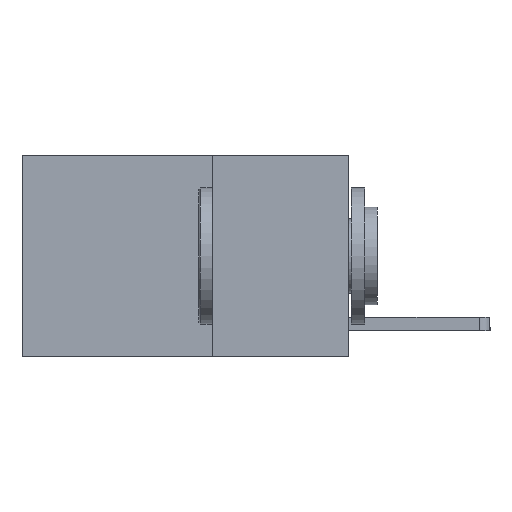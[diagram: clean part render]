
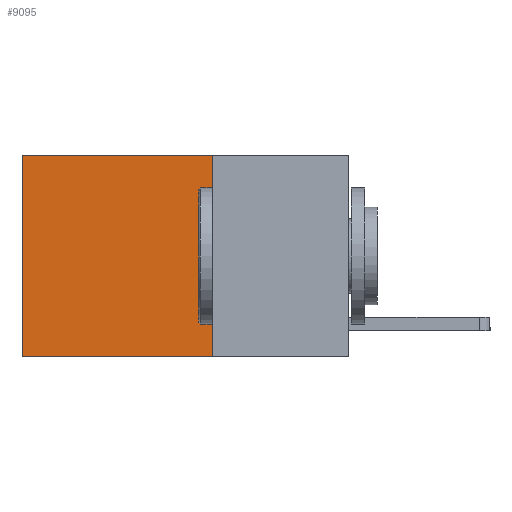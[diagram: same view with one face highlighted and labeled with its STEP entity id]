
A CAD part, left-side view. The second image highlights one B-rep face of the part: STEP entity #9095.
In plain terms, the highlighted planar face has unit normal (-1, 0, 0).
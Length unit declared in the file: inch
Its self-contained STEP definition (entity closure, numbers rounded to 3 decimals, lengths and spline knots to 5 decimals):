
#78 = VECTOR ( 'NONE', #3506, 39.37008 ) ;
#290 = EDGE_CURVE ( 'NONE', #3493, #10487, #9896, .T. ) ;
#1287 = ORIENTED_EDGE ( 'NONE', *, *, #3142, .T. ) ;
#1579 = AXIS2_PLACEMENT_3D ( 'NONE', #5952, #8208, #4128 ) ;
#2657 = VECTOR ( 'NONE', #7800, 39.37008 ) ;
#3085 = EDGE_LOOP ( 'NONE', ( #1287, #8092, #6186, #6902 ) ) ;
#3142 = EDGE_CURVE ( 'NONE', #10487, #8036, #9861, .T. ) ;
#3428 = PLANE ( 'NONE',  #1579 ) ;
#3493 = VERTEX_POINT ( 'NONE', #7069 ) ;
#3506 = DIRECTION ( 'NONE',  ( 0., 1., 0. ) ) ;
#4128 = DIRECTION ( 'NONE',  ( 0., 0., -1. ) ) ;
#4918 = VECTOR ( 'NONE', #6444, 39.37008 ) ;
#5848 = CARTESIAN_POINT ( 'NONE',  ( 0.2625, 0.6, 0. ) ) ;
#5952 = CARTESIAN_POINT ( 'NONE',  ( 0.2625, 0.25, 0. ) ) ;
#6030 = LINE ( 'NONE', #8283, #78 ) ;
#6059 = VERTEX_POINT ( 'NONE', #7624 ) ;
#6186 = ORIENTED_EDGE ( 'NONE', *, *, #6923, .F. ) ;
#6444 = DIRECTION ( 'NONE',  ( 0., 0., -1. ) ) ;
#6554 = FACE_OUTER_BOUND ( 'NONE', #3085, .T. ) ;
#6755 = EDGE_CURVE ( 'NONE', #6059, #8036, #6030, .T. ) ;
#6902 = ORIENTED_EDGE ( 'NONE', *, *, #290, .T. ) ;
#6923 = EDGE_CURVE ( 'NONE', #3493, #6059, #7045, .T. ) ;
#7045 = LINE ( 'NONE', #8597, #2657 ) ;
#7069 = CARTESIAN_POINT ( 'NONE',  ( 0.2625, 0.25, 0. ) ) ;
#7188 = CARTESIAN_POINT ( 'NONE',  ( 0.2625, 0.6, 0. ) ) ;
#7480 = DIRECTION ( 'NONE',  ( 0., 1., 0. ) ) ;
#7624 = CARTESIAN_POINT ( 'NONE',  ( 0.2625, 0.25, -0.37 ) ) ;
#7800 = DIRECTION ( 'NONE',  ( 0., 0., -1. ) ) ;
#8036 = VERTEX_POINT ( 'NONE', #10076 ) ;
#8092 = ORIENTED_EDGE ( 'NONE', *, *, #6755, .F. ) ;
#8208 = DIRECTION ( 'NONE',  ( 1., 0., 0. ) ) ;
#8283 = CARTESIAN_POINT ( 'NONE',  ( 0.2625, 0.25, -0.37 ) ) ;
#8597 = CARTESIAN_POINT ( 'NONE',  ( 0.2625, 0.25, 0. ) ) ;
#8698 = VECTOR ( 'NONE', #7480, 39.37008 ) ;
#9095 = ADVANCED_FACE ( 'NONE', ( #6554 ), #3428, .F. ) ;
#9847 = CARTESIAN_POINT ( 'NONE',  ( 0.2625, 0.25, 0. ) ) ;
#9861 = LINE ( 'NONE', #7188, #4918 ) ;
#9896 = LINE ( 'NONE', #9847, #8698 ) ;
#10076 = CARTESIAN_POINT ( 'NONE',  ( 0.2625, 0.6, -0.37 ) ) ;
#10487 = VERTEX_POINT ( 'NONE', #5848 ) ;
